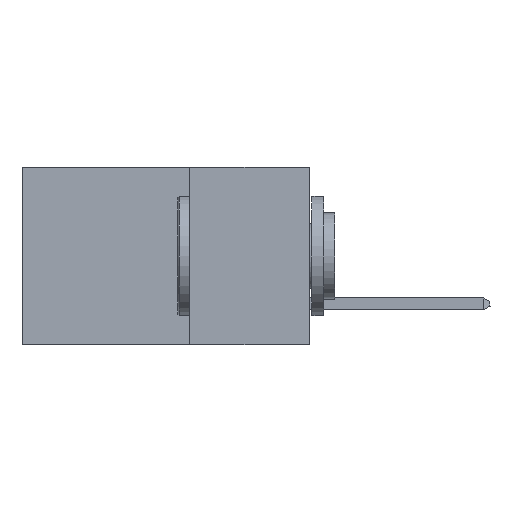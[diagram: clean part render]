
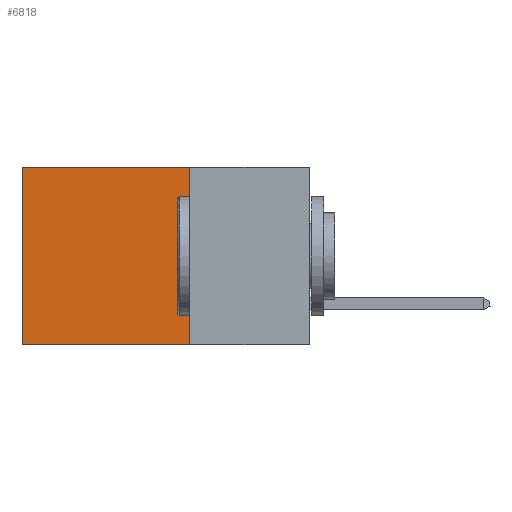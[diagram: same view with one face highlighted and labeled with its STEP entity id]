
A CAD part, left-side view. The second image highlights one B-rep face of the part: STEP entity #6818.
In plain terms, the highlighted planar face has unit normal (-1, 0, 0).
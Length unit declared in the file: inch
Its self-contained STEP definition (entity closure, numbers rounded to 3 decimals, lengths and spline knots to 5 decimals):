
#381 = ORIENTED_EDGE ( 'NONE', *, *, #15123, .F. ) ;
#1125 = CARTESIAN_POINT ( 'NONE',  ( 0.2875, 0.25, 0. ) ) ;
#1855 = LINE ( 'NONE', #12597, #10203 ) ;
#3642 = CARTESIAN_POINT ( 'NONE',  ( 0.2875, 0.25, 0. ) ) ;
#4458 = CARTESIAN_POINT ( 'NONE',  ( 0.2875, 0.25, -0.37 ) ) ;
#5244 = VERTEX_POINT ( 'NONE', #4458 ) ;
#5479 = EDGE_CURVE ( 'NONE', #15168, #8278, #17048, .T. ) ;
#5486 = ORIENTED_EDGE ( 'NONE', *, *, #5479, .T. ) ;
#5661 = EDGE_LOOP ( 'NONE', ( #20209, #381, #18650, #5486 ) ) ;
#5924 = CARTESIAN_POINT ( 'NONE',  ( 0.2875, 0.6, 0. ) ) ;
#6818 = ADVANCED_FACE ( 'NONE', ( #16770 ), #18179, .F. ) ;
#6927 = DIRECTION ( 'NONE',  ( 1., 0., 0. ) ) ;
#8278 = VERTEX_POINT ( 'NONE', #5924 ) ;
#8924 = VERTEX_POINT ( 'NONE', #19266 ) ;
#8948 = DIRECTION ( 'NONE',  ( 0., 0., -1. ) ) ;
#9013 = VECTOR ( 'NONE', #8948, 39.37008 ) ;
#10203 = VECTOR ( 'NONE', #20573, 39.37008 ) ;
#10286 = DIRECTION ( 'NONE',  ( 0., 1., 0. ) ) ;
#10806 = LINE ( 'NONE', #12607, #14536 ) ;
#11990 = EDGE_CURVE ( 'NONE', #15168, #5244, #1855, .T. ) ;
#12245 = VECTOR ( 'NONE', #10286, 39.37008 ) ;
#12597 = CARTESIAN_POINT ( 'NONE',  ( 0.2875, 0.25, 0. ) ) ;
#12607 = CARTESIAN_POINT ( 'NONE',  ( 0.2875, 0.25, -0.37 ) ) ;
#14214 = DIRECTION ( 'NONE',  ( 0., 1., 0. ) ) ;
#14536 = VECTOR ( 'NONE', #14214, 39.37008 ) ;
#14961 = EDGE_CURVE ( 'NONE', #8278, #8924, #18098, .T. ) ;
#15123 = EDGE_CURVE ( 'NONE', #5244, #8924, #10806, .T. ) ;
#15168 = VERTEX_POINT ( 'NONE', #1125 ) ;
#16770 = FACE_OUTER_BOUND ( 'NONE', #5661, .T. ) ;
#17048 = LINE ( 'NONE', #3642, #12245 ) ;
#17315 = AXIS2_PLACEMENT_3D ( 'NONE', #19690, #6927, #18239 ) ;
#18098 = LINE ( 'NONE', #20167, #9013 ) ;
#18179 = PLANE ( 'NONE',  #17315 ) ;
#18239 = DIRECTION ( 'NONE',  ( 0., 0., -1. ) ) ;
#18650 = ORIENTED_EDGE ( 'NONE', *, *, #11990, .F. ) ;
#19266 = CARTESIAN_POINT ( 'NONE',  ( 0.2875, 0.6, -0.37 ) ) ;
#19690 = CARTESIAN_POINT ( 'NONE',  ( 0.2875, 0.25, 0. ) ) ;
#20167 = CARTESIAN_POINT ( 'NONE',  ( 0.2875, 0.6, 0. ) ) ;
#20209 = ORIENTED_EDGE ( 'NONE', *, *, #14961, .T. ) ;
#20573 = DIRECTION ( 'NONE',  ( 0., 0., -1. ) ) ;
